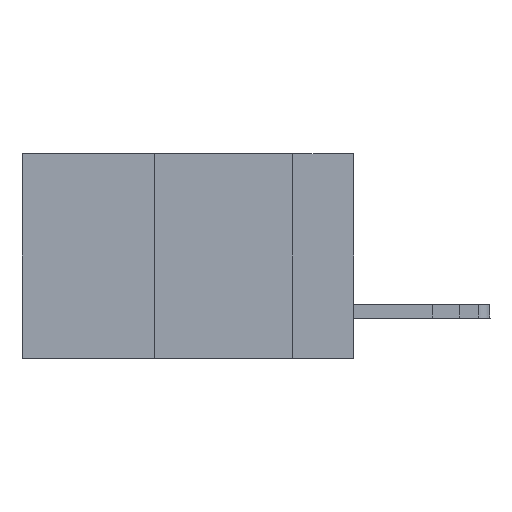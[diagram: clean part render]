
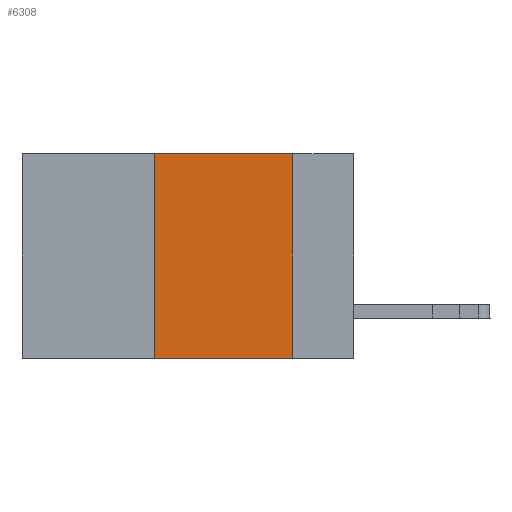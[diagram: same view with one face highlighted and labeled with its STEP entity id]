
A CAD part, left-side view. The second image highlights one B-rep face of the part: STEP entity #6308.
In plain terms, the highlighted planar face has unit normal (-1, 0, 0).
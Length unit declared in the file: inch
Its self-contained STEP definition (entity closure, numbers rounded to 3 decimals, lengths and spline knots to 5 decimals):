
#66 = LINE ( 'NONE', #1924, #3180 ) ;
#665 = CARTESIAN_POINT ( 'NONE',  ( 0., 0.11, -0.37 ) ) ;
#1531 = VECTOR ( 'NONE', #24017, 39.37008 ) ;
#1924 = CARTESIAN_POINT ( 'NONE',  ( 0., 0.11, 0. ) ) ;
#3180 = VECTOR ( 'NONE', #14088, 39.37008 ) ;
#3797 = CARTESIAN_POINT ( 'NONE',  ( 0., 0.6, 0. ) ) ;
#3803 = AXIS2_PLACEMENT_3D ( 'NONE', #17830, #22286, #9914 ) ;
#4321 = VERTEX_POINT ( 'NONE', #10832 ) ;
#4731 = VERTEX_POINT ( 'NONE', #665 ) ;
#5519 = EDGE_CURVE ( 'NONE', #20943, #4731, #12086, .T. ) ;
#5860 = VERTEX_POINT ( 'NONE', #16006 ) ;
#5945 = PLANE ( 'NONE',  #3803 ) ;
#6219 = LINE ( 'NONE', #15992, #1531 ) ;
#6308 = ADVANCED_FACE ( 'NONE', ( #19796 ), #5945, .F. ) ;
#7745 = EDGE_LOOP ( 'NONE', ( #23533, #11417, #19312, #17774 ) ) ;
#9914 = DIRECTION ( 'NONE',  ( 0., 0., -1. ) ) ;
#10224 = CARTESIAN_POINT ( 'NONE',  ( 0., 0.6, -0.37 ) ) ;
#10832 = CARTESIAN_POINT ( 'NONE',  ( 0., 0.36, 0. ) ) ;
#11417 = ORIENTED_EDGE ( 'NONE', *, *, #11760, .F. ) ;
#11760 = EDGE_CURVE ( 'NONE', #4321, #5860, #23574, .T. ) ;
#11877 = DIRECTION ( 'NONE',  ( 0., -1., 0. ) ) ;
#12086 = LINE ( 'NONE', #10224, #12637 ) ;
#12478 = DIRECTION ( 'NONE',  ( 0., -1., 0. ) ) ;
#12637 = VECTOR ( 'NONE', #12478, 39.37008 ) ;
#13244 = VECTOR ( 'NONE', #11877, 39.37008 ) ;
#14088 = DIRECTION ( 'NONE',  ( 0., 0., -1. ) ) ;
#15992 = CARTESIAN_POINT ( 'NONE',  ( 0., 0.36, 0. ) ) ;
#16006 = CARTESIAN_POINT ( 'NONE',  ( 0., 0.11, 0. ) ) ;
#17319 = EDGE_CURVE ( 'NONE', #5860, #4731, #66, .T. ) ;
#17774 = ORIENTED_EDGE ( 'NONE', *, *, #5519, .T. ) ;
#17830 = CARTESIAN_POINT ( 'NONE',  ( 0., 0.6, 0. ) ) ;
#18224 = EDGE_CURVE ( 'NONE', #20943, #4321, #6219, .T. ) ;
#19312 = ORIENTED_EDGE ( 'NONE', *, *, #18224, .F. ) ;
#19796 = FACE_OUTER_BOUND ( 'NONE', #7745, .T. ) ;
#20943 = VERTEX_POINT ( 'NONE', #25829 ) ;
#22286 = DIRECTION ( 'NONE',  ( 1., 0., 0. ) ) ;
#23533 = ORIENTED_EDGE ( 'NONE', *, *, #17319, .F. ) ;
#23574 = LINE ( 'NONE', #3797, #13244 ) ;
#24017 = DIRECTION ( 'NONE',  ( 0., 0., 1. ) ) ;
#25829 = CARTESIAN_POINT ( 'NONE',  ( 0., 0.36, -0.37 ) ) ;
